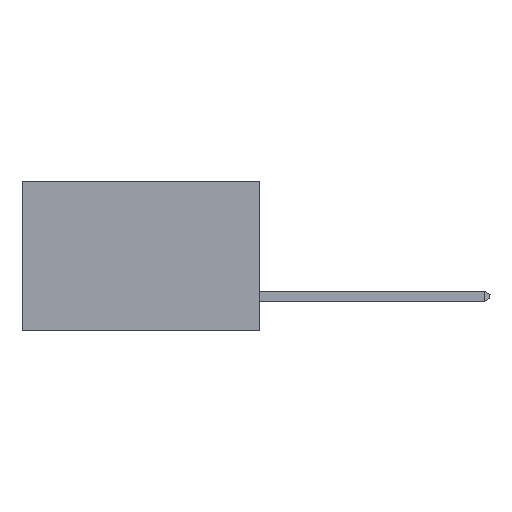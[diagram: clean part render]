
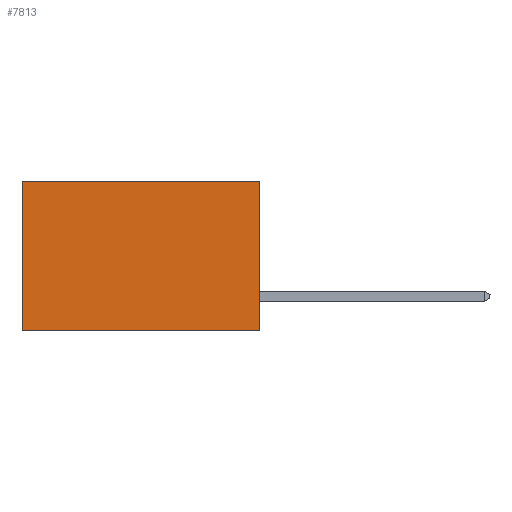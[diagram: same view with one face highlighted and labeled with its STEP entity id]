
A CAD part, left-side view. The second image highlights one B-rep face of the part: STEP entity #7813.
In plain terms, the highlighted planar face has unit normal (-1, 0, 0).
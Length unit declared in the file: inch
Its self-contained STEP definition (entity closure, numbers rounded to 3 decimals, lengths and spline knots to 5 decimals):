
#234 = ORIENTED_EDGE ( 'NONE', *, *, #700, .F. ) ;
#500 = EDGE_CURVE ( 'NONE', #3432, #3766, #4471, .T. ) ;
#700 = EDGE_CURVE ( 'NONE', #2814, #3432, #3896, .T. ) ;
#813 = DIRECTION ( 'NONE',  ( 0., 1., 0. ) ) ;
#965 = DIRECTION ( 'NONE',  ( 1., 0., 0. ) ) ;
#1305 = CARTESIAN_POINT ( 'NONE',  ( 0.277, 0., -0.37 ) ) ;
#1659 = CARTESIAN_POINT ( 'NONE',  ( 0.277, 0., 0. ) ) ;
#1870 = CARTESIAN_POINT ( 'NONE',  ( 0.277, 0.59, -0.37 ) ) ;
#1969 = CARTESIAN_POINT ( 'NONE',  ( 0.277, 0., 0. ) ) ;
#2277 = VERTEX_POINT ( 'NONE', #7263 ) ;
#2573 = PLANE ( 'NONE',  #3463 ) ;
#2647 = EDGE_CURVE ( 'NONE', #2814, #2277, #8606, .T. ) ;
#2757 = VECTOR ( 'NONE', #7019, 39.37008 ) ;
#2814 = VERTEX_POINT ( 'NONE', #1659 ) ;
#2918 = ORIENTED_EDGE ( 'NONE', *, *, #2647, .T. ) ;
#3263 = EDGE_CURVE ( 'NONE', #2277, #3766, #8910, .T. ) ;
#3432 = VERTEX_POINT ( 'NONE', #8109 ) ;
#3463 = AXIS2_PLACEMENT_3D ( 'NONE', #4787, #965, #6113 ) ;
#3766 = VERTEX_POINT ( 'NONE', #5439 ) ;
#3896 = LINE ( 'NONE', #6290, #7195 ) ;
#3947 = VECTOR ( 'NONE', #7603, 39.37008 ) ;
#4471 = LINE ( 'NONE', #1305, #2757 ) ;
#4787 = CARTESIAN_POINT ( 'NONE',  ( 0.277, 0., -0.37 ) ) ;
#5260 = DIRECTION ( 'NONE',  ( 0., 0., -1. ) ) ;
#5439 = CARTESIAN_POINT ( 'NONE',  ( 0.277, 0.59, -0.37 ) ) ;
#5579 = ORIENTED_EDGE ( 'NONE', *, *, #3263, .T. ) ;
#5782 = ORIENTED_EDGE ( 'NONE', *, *, #500, .F. ) ;
#6113 = DIRECTION ( 'NONE',  ( 0., 0., -1. ) ) ;
#6290 = CARTESIAN_POINT ( 'NONE',  ( 0.277, 0., -0.37 ) ) ;
#7019 = DIRECTION ( 'NONE',  ( 0., 1., 0. ) ) ;
#7076 = VECTOR ( 'NONE', #813, 39.37008 ) ;
#7195 = VECTOR ( 'NONE', #5260, 39.37008 ) ;
#7263 = CARTESIAN_POINT ( 'NONE',  ( 0.277, 0.59, 0. ) ) ;
#7603 = DIRECTION ( 'NONE',  ( 0., 0., -1. ) ) ;
#7813 = ADVANCED_FACE ( 'NONE', ( #8008 ), #2573, .F. ) ;
#8008 = FACE_OUTER_BOUND ( 'NONE', #8543, .T. ) ;
#8109 = CARTESIAN_POINT ( 'NONE',  ( 0.277, 0., -0.37 ) ) ;
#8543 = EDGE_LOOP ( 'NONE', ( #5579, #5782, #234, #2918 ) ) ;
#8606 = LINE ( 'NONE', #1969, #7076 ) ;
#8910 = LINE ( 'NONE', #1870, #3947 ) ;
